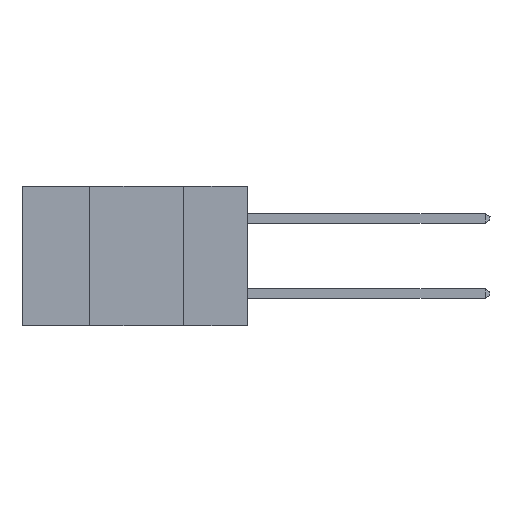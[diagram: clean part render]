
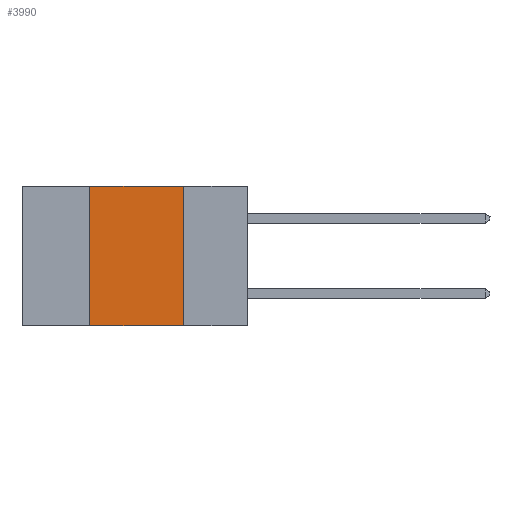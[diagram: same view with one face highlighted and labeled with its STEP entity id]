
A CAD part, left-side view. The second image highlights one B-rep face of the part: STEP entity #3990.
In plain terms, the highlighted planar face has unit normal (-1, 0, 0).
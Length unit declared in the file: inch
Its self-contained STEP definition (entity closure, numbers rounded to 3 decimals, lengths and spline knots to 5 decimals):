
#1412 = EDGE_LOOP ( 'NONE', ( #8049, #14915, #14138, #11925 ) ) ;
#3561 = PLANE ( 'NONE',  #22824 ) ;
#3990 = ADVANCED_FACE ( 'NONE', ( #12601 ), #3561, .F. ) ;
#4609 = LINE ( 'NONE', #12380, #4668 ) ;
#4668 = VECTOR ( 'NONE', #8445, 39.37008 ) ;
#5152 = CARTESIAN_POINT ( 'NONE',  ( 0., 0.17, -0.37 ) ) ;
#5941 = VERTEX_POINT ( 'NONE', #7909 ) ;
#6015 = EDGE_CURVE ( 'NONE', #9184, #5941, #26502, .T. ) ;
#6983 = VECTOR ( 'NONE', #10073, 39.37008 ) ;
#7188 = CARTESIAN_POINT ( 'NONE',  ( 0., 0.17, 0. ) ) ;
#7617 = LINE ( 'NONE', #5152, #19108 ) ;
#7891 = EDGE_CURVE ( 'NONE', #13422, #5941, #7617, .T. ) ;
#7909 = CARTESIAN_POINT ( 'NONE',  ( 0., 0.17, -0.37 ) ) ;
#8049 = ORIENTED_EDGE ( 'NONE', *, *, #7891, .F. ) ;
#8445 = DIRECTION ( 'NONE',  ( 0., -1., 0. ) ) ;
#9184 = VERTEX_POINT ( 'NONE', #15307 ) ;
#10073 = DIRECTION ( 'NONE',  ( 0., -1., 0. ) ) ;
#11526 = DIRECTION ( 'NONE',  ( 0., 0., -1. ) ) ;
#11528 = DIRECTION ( 'NONE',  ( 0., 0., 1. ) ) ;
#11925 = ORIENTED_EDGE ( 'NONE', *, *, #6015, .T. ) ;
#12380 = CARTESIAN_POINT ( 'NONE',  ( 0., 0.6, 0. ) ) ;
#12601 = FACE_OUTER_BOUND ( 'NONE', #1412, .T. ) ;
#13422 = VERTEX_POINT ( 'NONE', #7188 ) ;
#14005 = CARTESIAN_POINT ( 'NONE',  ( 0., 0.6, 0. ) ) ;
#14138 = ORIENTED_EDGE ( 'NONE', *, *, #20113, .F. ) ;
#14915 = ORIENTED_EDGE ( 'NONE', *, *, #17522, .F. ) ;
#15055 = LINE ( 'NONE', #17237, #22917 ) ;
#15307 = CARTESIAN_POINT ( 'NONE',  ( 0., 0.42, -0.37 ) ) ;
#16169 = CARTESIAN_POINT ( 'NONE',  ( 0., 0.6, -0.37 ) ) ;
#17237 = CARTESIAN_POINT ( 'NONE',  ( 0., 0.42, -0.37 ) ) ;
#17522 = EDGE_CURVE ( 'NONE', #21899, #13422, #4609, .T. ) ;
#19108 = VECTOR ( 'NONE', #11526, 39.37008 ) ;
#19975 = DIRECTION ( 'NONE',  ( 1., 0., 0. ) ) ;
#20113 = EDGE_CURVE ( 'NONE', #9184, #21899, #15055, .T. ) ;
#20243 = DIRECTION ( 'NONE',  ( 0., 0., -1. ) ) ;
#21899 = VERTEX_POINT ( 'NONE', #23600 ) ;
#22824 = AXIS2_PLACEMENT_3D ( 'NONE', #14005, #19975, #20243 ) ;
#22917 = VECTOR ( 'NONE', #11528, 39.37008 ) ;
#23600 = CARTESIAN_POINT ( 'NONE',  ( 0., 0.42, 0. ) ) ;
#26502 = LINE ( 'NONE', #16169, #6983 ) ;
